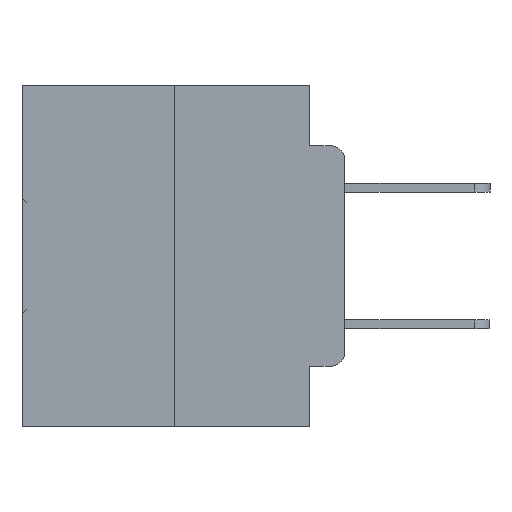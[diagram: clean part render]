
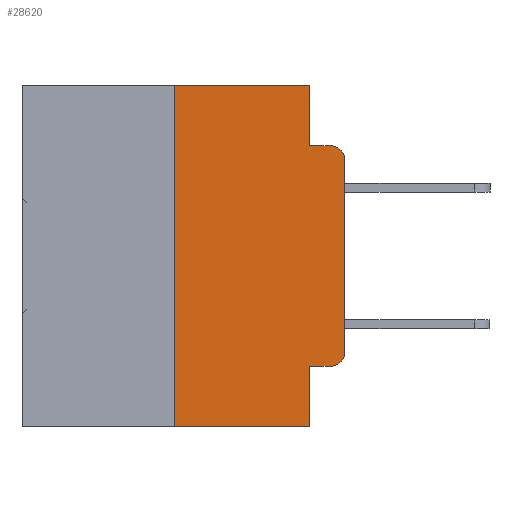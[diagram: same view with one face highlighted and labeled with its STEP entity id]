
A CAD part, left-side view. The second image highlights one B-rep face of the part: STEP entity #28620.
In plain terms, the highlighted planar face has unit normal (-1, 0, 0).
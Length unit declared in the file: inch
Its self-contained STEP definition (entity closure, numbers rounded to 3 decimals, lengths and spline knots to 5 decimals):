
#348 = VECTOR ( 'NONE', #2333, 39.37008 ) ;
#471 = EDGE_CURVE ( 'NONE', #5710, #21650, #15304, .T. ) ;
#1182 = LINE ( 'NONE', #15640, #348 ) ;
#1230 = LINE ( 'NONE', #14198, #5858 ) ;
#1575 = VERTEX_POINT ( 'NONE', #14676 ) ;
#1685 = DIRECTION ( 'NONE',  ( 0., -1., 0. ) ) ;
#2211 = EDGE_CURVE ( 'NONE', #5710, #33358, #11438, .T. ) ;
#2282 = DIRECTION ( 'NONE',  ( -1., 0., 0. ) ) ;
#2333 = DIRECTION ( 'NONE',  ( 0., 0., 1. ) ) ;
#3651 = CARTESIAN_POINT ( 'NONE',  ( 0., 0.25, -0.5 ) ) ;
#3965 = EDGE_CURVE ( 'NONE', #30138, #1575, #1230, .T. ) ;
#4296 = CARTESIAN_POINT ( 'NONE',  ( 0., 0.473, -0.5 ) ) ;
#4409 = CARTESIAN_POINT ( 'NONE',  ( 0., 0.051, -0.4115 ) ) ;
#5141 = AXIS2_PLACEMENT_3D ( 'NONE', #27334, #32632, #16938 ) ;
#5710 = VERTEX_POINT ( 'NONE', #25679 ) ;
#5858 = VECTOR ( 'NONE', #1685, 39.37008 ) ;
#5879 = LINE ( 'NONE', #13147, #19181 ) ;
#6801 = DIRECTION ( 'NONE',  ( 0., -1., 0. ) ) ;
#7268 = CARTESIAN_POINT ( 'NONE',  ( 0., 0.051, -0.0885 ) ) ;
#7555 = VERTEX_POINT ( 'NONE', #7774 ) ;
#7774 = CARTESIAN_POINT ( 'NONE',  ( 0., 0.25, 0. ) ) ;
#7785 = ORIENTED_EDGE ( 'NONE', *, *, #21738, .T. ) ;
#7800 = VERTEX_POINT ( 'NONE', #14085 ) ;
#8206 = VECTOR ( 'NONE', #32453, 39.37008 ) ;
#9185 = AXIS2_PLACEMENT_3D ( 'NONE', #18247, #2282, #20887 ) ;
#9239 = VERTEX_POINT ( 'NONE', #33369 ) ;
#9269 = EDGE_CURVE ( 'NONE', #33358, #9239, #19157, .T. ) ;
#11360 = VERTEX_POINT ( 'NONE', #20306 ) ;
#11438 = LINE ( 'NONE', #4409, #18475 ) ;
#11921 = CIRCLE ( 'NONE', #9185, 0.02 ) ;
#12150 = DIRECTION ( 'NONE',  ( 0., -1., 0. ) ) ;
#12512 = CARTESIAN_POINT ( 'NONE',  ( 0., 0.051, 0. ) ) ;
#12581 = CARTESIAN_POINT ( 'NONE',  ( 0., 0.02, -0.4115 ) ) ;
#12950 = EDGE_CURVE ( 'NONE', #7800, #1575, #11921, .T. ) ;
#13145 = EDGE_LOOP ( 'NONE', ( #7785, #21898, #31224, #30786, #27291, #33950, #27757, #19376, #33070, #20368 ) ) ;
#13147 = CARTESIAN_POINT ( 'NONE',  ( 0., 0.473, 0. ) ) ;
#14085 = CARTESIAN_POINT ( 'NONE',  ( 0., 0., -0.1085 ) ) ;
#14198 = CARTESIAN_POINT ( 'NONE',  ( 0., 0.051, -0.0885 ) ) ;
#14676 = CARTESIAN_POINT ( 'NONE',  ( 0., 0.02, -0.0885 ) ) ;
#14794 = CARTESIAN_POINT ( 'NONE',  ( 0., 0.051, 0. ) ) ;
#15259 = DIRECTION ( 'NONE',  ( -1., 0., 0. ) ) ;
#15304 = LINE ( 'NONE', #12512, #8206 ) ;
#15640 = CARTESIAN_POINT ( 'NONE',  ( 0., 0.25, 0. ) ) ;
#15953 = VECTOR ( 'NONE', #12150, 39.37008 ) ;
#16399 = CARTESIAN_POINT ( 'NONE',  ( 0., 0.051, -0.5 ) ) ;
#16927 = LINE ( 'NONE', #24564, #29995 ) ;
#16938 = DIRECTION ( 'NONE',  ( 0., 0., -1. ) ) ;
#17456 = DIRECTION ( 'NONE',  ( 0., 0., -1. ) ) ;
#18247 = CARTESIAN_POINT ( 'NONE',  ( 0., 0.02, -0.1085 ) ) ;
#18428 = LINE ( 'NONE', #4296, #15953 ) ;
#18475 = VECTOR ( 'NONE', #6801, 39.37008 ) ;
#18880 = EDGE_CURVE ( 'NONE', #27314, #7555, #1182, .T. ) ;
#19157 = CIRCLE ( 'NONE', #33122, 0.02 ) ;
#19181 = VECTOR ( 'NONE', #34099, 39.37008 ) ;
#19253 = LINE ( 'NONE', #14794, #32359 ) ;
#19376 = ORIENTED_EDGE ( 'NONE', *, *, #471, .F. ) ;
#20306 = CARTESIAN_POINT ( 'NONE',  ( 0., 0.051, 0. ) ) ;
#20368 = ORIENTED_EDGE ( 'NONE', *, *, #9269, .T. ) ;
#20887 = DIRECTION ( 'NONE',  ( 0., 0., -1. ) ) ;
#21650 = VERTEX_POINT ( 'NONE', #16399 ) ;
#21738 = EDGE_CURVE ( 'NONE', #9239, #7800, #16927, .T. ) ;
#21810 = FACE_OUTER_BOUND ( 'NONE', #13145, .T. ) ;
#21898 = ORIENTED_EDGE ( 'NONE', *, *, #12950, .T. ) ;
#23990 = EDGE_CURVE ( 'NONE', #27314, #21650, #18428, .T. ) ;
#24564 = CARTESIAN_POINT ( 'NONE',  ( 0., 0., 0. ) ) ;
#25679 = CARTESIAN_POINT ( 'NONE',  ( 0., 0.051, -0.4115 ) ) ;
#27160 = DIRECTION ( 'NONE',  ( 0., 0., 1. ) ) ;
#27291 = ORIENTED_EDGE ( 'NONE', *, *, #30288, .F. ) ;
#27314 = VERTEX_POINT ( 'NONE', #3651 ) ;
#27334 = CARTESIAN_POINT ( 'NONE',  ( 0., 0.473, 0. ) ) ;
#27757 = ORIENTED_EDGE ( 'NONE', *, *, #23990, .T. ) ;
#28620 = ADVANCED_FACE ( 'NONE', ( #21810 ), #32511, .F. ) ;
#29383 = EDGE_CURVE ( 'NONE', #11360, #30138, #19253, .T. ) ;
#29995 = VECTOR ( 'NONE', #27160, 39.37008 ) ;
#30138 = VERTEX_POINT ( 'NONE', #7268 ) ;
#30288 = EDGE_CURVE ( 'NONE', #7555, #11360, #5879, .T. ) ;
#30786 = ORIENTED_EDGE ( 'NONE', *, *, #29383, .F. ) ;
#30946 = CARTESIAN_POINT ( 'NONE',  ( 0., 0.02, -0.3915 ) ) ;
#31224 = ORIENTED_EDGE ( 'NONE', *, *, #3965, .F. ) ;
#32359 = VECTOR ( 'NONE', #17456, 39.37008 ) ;
#32453 = DIRECTION ( 'NONE',  ( 0., 0., -1. ) ) ;
#32511 = PLANE ( 'NONE',  #5141 ) ;
#32632 = DIRECTION ( 'NONE',  ( 1., 0., 0. ) ) ;
#33070 = ORIENTED_EDGE ( 'NONE', *, *, #2211, .T. ) ;
#33122 = AXIS2_PLACEMENT_3D ( 'NONE', #30946, #15259, #33596 ) ;
#33358 = VERTEX_POINT ( 'NONE', #12581 ) ;
#33369 = CARTESIAN_POINT ( 'NONE',  ( 0., 0., -0.3915 ) ) ;
#33596 = DIRECTION ( 'NONE',  ( 0., 0., -1. ) ) ;
#33950 = ORIENTED_EDGE ( 'NONE', *, *, #18880, .F. ) ;
#34099 = DIRECTION ( 'NONE',  ( 0., -1., 0. ) ) ;
